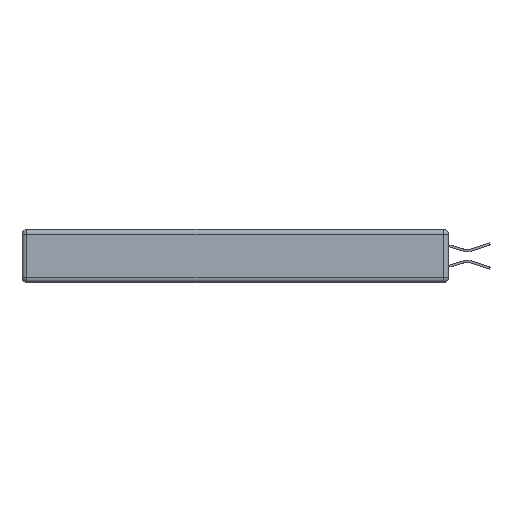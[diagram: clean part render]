
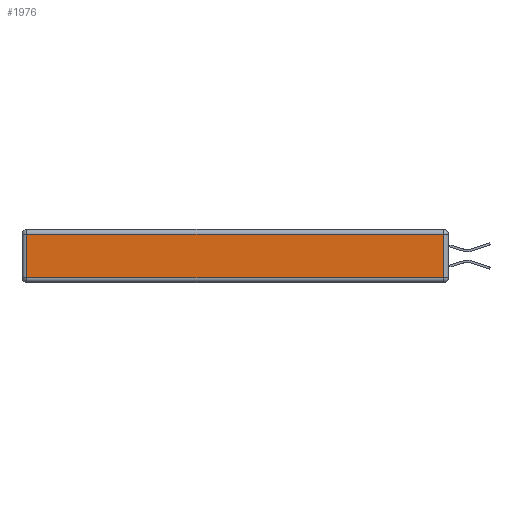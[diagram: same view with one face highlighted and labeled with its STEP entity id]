
A CAD part, left-side view. The second image highlights one B-rep face of the part: STEP entity #1976.
In plain terms, the highlighted planar face has unit normal (-1, 0, 0).
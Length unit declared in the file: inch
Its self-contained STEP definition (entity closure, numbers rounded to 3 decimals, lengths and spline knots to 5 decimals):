
#25 = EDGE_CURVE ( 'NONE', #10720, #8380, #6636, .T. ) ;
#114 = EDGE_CURVE ( 'NONE', #8380, #8058, #13270, .T. ) ;
#154 = CARTESIAN_POINT ( 'NONE',  ( 0., 0.03, -0.313 ) ) ;
#263 = ORIENTED_EDGE ( 'NONE', *, *, #14263, .T. ) ;
#320 = CARTESIAN_POINT ( 'NONE',  ( 0., 2.72, -0.03 ) ) ;
#773 = LINE ( 'NONE', #2026, #10394 ) ;
#1769 = DIRECTION ( 'NONE',  ( 0., 0., 1. ) ) ;
#1976 = ADVANCED_FACE ( 'NONE', ( #5094 ), #2065, .T. ) ;
#2026 = CARTESIAN_POINT ( 'NONE',  ( 0., 2.72, -0.343 ) ) ;
#2065 = PLANE ( 'NONE',  #10567 ) ;
#3165 = CARTESIAN_POINT ( 'NONE',  ( 0., 2.75, -0.03 ) ) ;
#4927 = EDGE_CURVE ( 'NONE', #8058, #10291, #773, .T. ) ;
#5094 = FACE_OUTER_BOUND ( 'NONE', #11536, .T. ) ;
#6081 = VECTOR ( 'NONE', #1769, 39.37008 ) ;
#6636 = LINE ( 'NONE', #13378, #6081 ) ;
#6688 = CARTESIAN_POINT ( 'NONE',  ( 0., 0., -0.343 ) ) ;
#6747 = LINE ( 'NONE', #11690, #14856 ) ;
#6998 = VECTOR ( 'NONE', #8893, 39.37008 ) ;
#8058 = VERTEX_POINT ( 'NONE', #320 ) ;
#8380 = VERTEX_POINT ( 'NONE', #13880 ) ;
#8893 = DIRECTION ( 'NONE',  ( 0., 1., 0. ) ) ;
#9990 = CARTESIAN_POINT ( 'NONE',  ( 0., 2.72, -0.313 ) ) ;
#10291 = VERTEX_POINT ( 'NONE', #9990 ) ;
#10394 = VECTOR ( 'NONE', #14872, 39.37008 ) ;
#10567 = AXIS2_PLACEMENT_3D ( 'NONE', #6688, #14766, #11484 ) ;
#10720 = VERTEX_POINT ( 'NONE', #154 ) ;
#11252 = ORIENTED_EDGE ( 'NONE', *, *, #114, .T. ) ;
#11484 = DIRECTION ( 'NONE',  ( 0., 0., 1. ) ) ;
#11536 = EDGE_LOOP ( 'NONE', ( #263, #11884, #11252, #14164 ) ) ;
#11690 = CARTESIAN_POINT ( 'NONE',  ( 0., 0., -0.313 ) ) ;
#11747 = DIRECTION ( 'NONE',  ( 0., -1., 0. ) ) ;
#11884 = ORIENTED_EDGE ( 'NONE', *, *, #25, .T. ) ;
#13270 = LINE ( 'NONE', #3165, #6998 ) ;
#13378 = CARTESIAN_POINT ( 'NONE',  ( 0., 0.03, -0.343 ) ) ;
#13880 = CARTESIAN_POINT ( 'NONE',  ( 0., 0.03, -0.03 ) ) ;
#14164 = ORIENTED_EDGE ( 'NONE', *, *, #4927, .T. ) ;
#14263 = EDGE_CURVE ( 'NONE', #10291, #10720, #6747, .T. ) ;
#14766 = DIRECTION ( 'NONE',  ( -1., 0., 0. ) ) ;
#14856 = VECTOR ( 'NONE', #11747, 39.37008 ) ;
#14872 = DIRECTION ( 'NONE',  ( 0., 0., -1. ) ) ;
